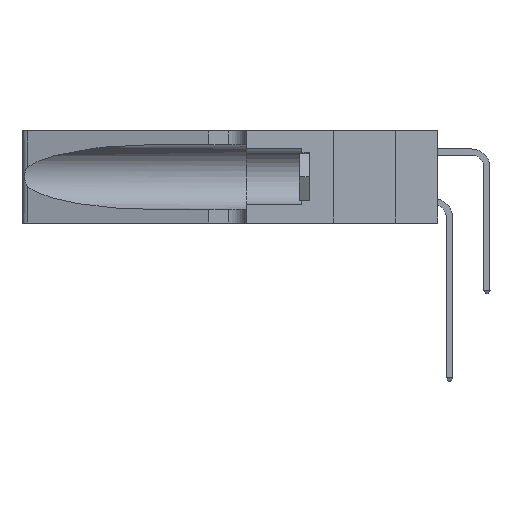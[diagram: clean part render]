
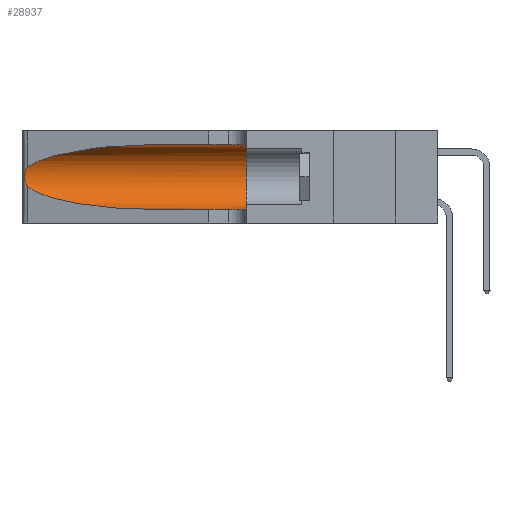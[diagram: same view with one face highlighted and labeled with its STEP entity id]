
A CAD part, left-side view. The second image highlights one B-rep face of the part: STEP entity #28937.
In plain terms, the highlighted cylindrical face has radius 3.308 mm (diameter 6.617 mm), a partial arc.
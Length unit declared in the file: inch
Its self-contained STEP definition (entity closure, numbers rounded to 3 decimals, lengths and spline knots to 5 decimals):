
#862 = CYLINDRICAL_SURFACE ( 'NONE', #14816, 0.13025 ) ;
#1482 = DIRECTION ( 'NONE',  ( 0., -1., 0. ) ) ;
#1985 = CARTESIAN_POINT ( 'NONE',  ( 0.25787, 1.23484, 0.2124 ) ) ;
#2080 = EDGE_CURVE ( 'NONE', #29145, #14054, #25563, .T. ) ;
#2238 = CARTESIAN_POINT ( 'NONE',  ( 0.18966, 0.96281, 0.31525 ) ) ;
#3040 = ORIENTED_EDGE ( 'NONE', *, *, #15029, .T. ) ;
#3365 = EDGE_CURVE ( 'NONE', #31393, #21157, #10554, .T. ) ;
#4249 = CARTESIAN_POINT ( 'NONE',  ( 0.26075, 1.23896, 0.178 ) ) ;
#4482 = CARTESIAN_POINT ( 'NONE',  ( 0.26018, 1.23835, 0.19895 ) ) ;
#4503 = VECTOR ( 'NONE', #33317, 39.37008 ) ;
#6582 = DIRECTION ( 'NONE',  ( 0., 0., 1. ) ) ;
#6662 = CARTESIAN_POINT ( 'NONE',  ( 0.25487, 1.22718, 0.14631 ) ) ;
#7106 = CARTESIAN_POINT ( 'NONE',  ( 0.1305, 0.72297, 0.05475 ) ) ;
#7482 = CARTESIAN_POINT ( 'NONE',  ( 0.1305, 0.72297, 0.31525 ) ) ;
#8208 = LINE ( 'NONE', #27484, #28620 ) ;
#8955 = VERTEX_POINT ( 'NONE', #9603 ) ;
#9257 = CARTESIAN_POINT ( 'NONE',  ( 0.25854, 1.2359, 0.20912 ) ) ;
#9495 = CARTESIAN_POINT ( 'NONE',  ( 0.25639, 1.23186, 0.15144 ) ) ;
#9535 = CARTESIAN_POINT ( 'NONE',  ( 0.1305, 0.35, 0.185 ) ) ;
#9603 = CARTESIAN_POINT ( 'NONE',  ( 0.25487, 1.22718, 0.14631 ) ) ;
#9739 = CARTESIAN_POINT ( 'NONE',  ( 0.26075, 1.23896, 0.19203 ) ) ;
#9815 = CARTESIAN_POINT ( 'NONE',  ( 0.1305, 1.61858, 0.05475 ) ) ;
#10341 = EDGE_CURVE ( 'NONE', #8955, #30147, #30169, .T. ) ;
#10554 = CIRCLE ( 'NONE', #15057, 0.13025 ) ;
#10817 = CARTESIAN_POINT ( 'NONE',  ( 0.1305, 0.35, 0.05475 ) ) ;
#11739 = ORIENTED_EDGE ( 'NONE', *, *, #14093, .F. ) ;
#11898 = CARTESIAN_POINT ( 'NONE',  ( 0.25555, 1.22994, 0.2215 ) ) ;
#12140 = CARTESIAN_POINT ( 'NONE',  ( 0.25487, 1.22718, 0.22369 ) ) ;
#12448 = CARTESIAN_POINT ( 'NONE',  ( 0.18966, 0.96281, 0.05475 ) ) ;
#13437 = B_SPLINE_CURVE_WITH_KNOTS ( 'NONE', 3,
 ( #12140, #11898, #22500, #1985, #9257, #4482, #9739, #4249, #17605, #30383, #14748, #9495, #17146, #6662 ),
 .UNSPECIFIED., .F., .F.,
 ( 4, 2, 2, 2, 2, 2, 4 ),
 ( 0., 0.00027, 0.00053, 0.00107, 0.0016, 0.00187, 0.00214 ),
 .UNSPECIFIED. ) ;
#14002 = DIRECTION ( 'NONE',  ( 0., -1., 0. ) ) ;
#14054 = VERTEX_POINT ( 'NONE', #21879 ) ;
#14093 = EDGE_CURVE ( 'NONE', #29145, #31393, #8208, .T. ) ;
#14748 = CARTESIAN_POINT ( 'NONE',  ( 0.25789, 1.23486, 0.15765 ) ) ;
#14752 = EDGE_CURVE ( 'NONE', #30147, #21157, #32994, .T. ) ;
#14816 = AXIS2_PLACEMENT_3D ( 'NONE', #21043, #14002, #27946 ) ;
#15029 = EDGE_CURVE ( 'NONE', #14054, #8955, #13437, .T. ) ;
#15057 = AXIS2_PLACEMENT_3D ( 'NONE', #9535, #19570, #6582 ) ;
#15118 = CARTESIAN_POINT ( 'NONE',  ( 0.2373, 1.15595, 0.28018 ) ) ;
#16162 = ORIENTED_EDGE ( 'NONE', *, *, #2080, .T. ) ;
#16995 = CARTESIAN_POINT ( 'NONE',  ( 0.1305, 0.72297, 0.31525 ) ) ;
#17146 = CARTESIAN_POINT ( 'NONE',  ( 0.25555, 1.22993, 0.14849 ) ) ;
#17605 = CARTESIAN_POINT ( 'NONE',  ( 0.26017, 1.23833, 0.17102 ) ) ;
#17746 = CARTESIAN_POINT ( 'NONE',  ( 0.25487, 1.22718, 0.22369 ) ) ;
#18413 = EDGE_LOOP ( 'NONE', ( #16162, #3040, #25253, #29048, #31088, #11739 ) ) ;
#19570 = DIRECTION ( 'NONE',  ( 0., 1., 0. ) ) ;
#20115 = FACE_OUTER_BOUND ( 'NONE', #18413, .T. ) ;
#20725 = CARTESIAN_POINT ( 'NONE',  ( 0.1305, 0.35, 0.31525 ) ) ;
#21043 = CARTESIAN_POINT ( 'NONE',  ( 0.1305, 1.61858, 0.185 ) ) ;
#21157 = VERTEX_POINT ( 'NONE', #10817 ) ;
#21879 = CARTESIAN_POINT ( 'NONE',  ( 0.25487, 1.22718, 0.22369 ) ) ;
#22500 = CARTESIAN_POINT ( 'NONE',  ( 0.25639, 1.23184, 0.21858 ) ) ;
#23127 = CARTESIAN_POINT ( 'NONE',  ( 0.2373, 1.15595, 0.08982 ) ) ;
#23208 = CARTESIAN_POINT ( 'NONE',  ( 0.1305, 0.72297, 0.05475 ) ) ;
#23909 = CARTESIAN_POINT ( 'NONE',  ( 0.25487, 1.22718, 0.14631 ) ) ;
#25253 = ORIENTED_EDGE ( 'NONE', *, *, #10341, .T. ) ;
#25563 =( BOUNDED_CURVE ( )  B_SPLINE_CURVE ( 3, ( #7482, #2238, #15118, #17746 ),
 .UNSPECIFIED., .F., .T. ) 
 B_SPLINE_CURVE_WITH_KNOTS ( ( 4, 4 ),
 ( 1.5708, 2.84003 ),
 .UNSPECIFIED. ) 
 CURVE ( )  GEOMETRIC_REPRESENTATION_ITEM ( )  RATIONAL_B_SPLINE_CURVE ( ( 1., 0.87, 0.87, 1. ) ) 
 REPRESENTATION_ITEM ( '' )  );
#27484 = CARTESIAN_POINT ( 'NONE',  ( 0.1305, 1.61858, 0.31525 ) ) ;
#27946 = DIRECTION ( 'NONE',  ( 0., 0., -1. ) ) ;
#28620 = VECTOR ( 'NONE', #1482, 39.37008 ) ;
#28937 = ADVANCED_FACE ( 'NONE', ( #20115 ), #862, .F. ) ;
#29048 = ORIENTED_EDGE ( 'NONE', *, *, #14752, .T. ) ;
#29145 = VERTEX_POINT ( 'NONE', #16995 ) ;
#30147 = VERTEX_POINT ( 'NONE', #23208 ) ;
#30169 =( BOUNDED_CURVE ( )  B_SPLINE_CURVE ( 3, ( #23909, #23127, #12448, #7106 ),
 .UNSPECIFIED., .F., .T. ) 
 B_SPLINE_CURVE_WITH_KNOTS ( ( 4, 4 ),
 ( 3.44316, 4.71239 ),
 .UNSPECIFIED. ) 
 CURVE ( )  GEOMETRIC_REPRESENTATION_ITEM ( )  RATIONAL_B_SPLINE_CURVE ( ( 1., 0.87, 0.87, 1. ) ) 
 REPRESENTATION_ITEM ( '' )  );
#30383 = CARTESIAN_POINT ( 'NONE',  ( 0.25856, 1.23593, 0.16098 ) ) ;
#31088 = ORIENTED_EDGE ( 'NONE', *, *, #3365, .F. ) ;
#31393 = VERTEX_POINT ( 'NONE', #20725 ) ;
#32994 = LINE ( 'NONE', #9815, #4503 ) ;
#33317 = DIRECTION ( 'NONE',  ( 0., -1., 0. ) ) ;
